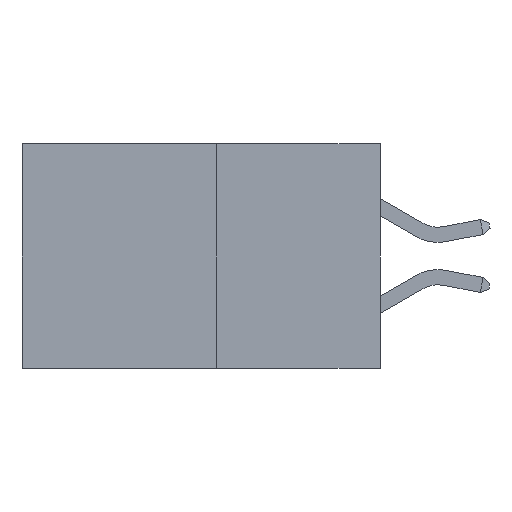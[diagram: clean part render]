
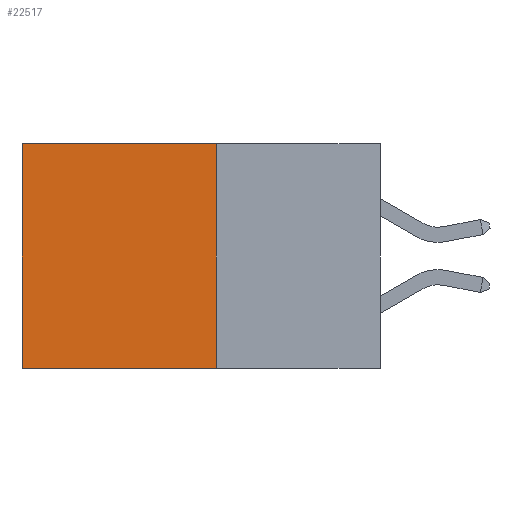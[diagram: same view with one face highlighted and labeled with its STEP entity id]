
A CAD part, left-side view. The second image highlights one B-rep face of the part: STEP entity #22517.
In plain terms, the highlighted planar face has unit normal (-1, 0, 0).
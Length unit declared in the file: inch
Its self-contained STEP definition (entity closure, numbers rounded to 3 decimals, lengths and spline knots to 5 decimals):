
#89 = LINE ( 'NONE', #22665, #4940 ) ;
#749 = EDGE_CURVE ( 'NONE', #18673, #10281, #4809, .T. ) ;
#1871 = ORIENTED_EDGE ( 'NONE', *, *, #24266, .F. ) ;
#1953 = DIRECTION ( 'NONE',  ( 0., 1., 0. ) ) ;
#2488 = CARTESIAN_POINT ( 'NONE',  ( 0.277, 0.27, -0.37 ) ) ;
#2747 = CARTESIAN_POINT ( 'NONE',  ( 0.277, 0.59, -0.37 ) ) ;
#3025 = EDGE_LOOP ( 'NONE', ( #8569, #1871, #23358, #18599 ) ) ;
#4348 = EDGE_CURVE ( 'NONE', #9320, #18673, #89, .T. ) ;
#4773 = VERTEX_POINT ( 'NONE', #17671 ) ;
#4809 = LINE ( 'NONE', #6474, #10126 ) ;
#4938 = DIRECTION ( 'NONE',  ( 0., 0., -1. ) ) ;
#4940 = VECTOR ( 'NONE', #22587, 39.37008 ) ;
#5736 = FACE_OUTER_BOUND ( 'NONE', #3025, .T. ) ;
#5994 = AXIS2_PLACEMENT_3D ( 'NONE', #2488, #16429, #4938 ) ;
#6474 = CARTESIAN_POINT ( 'NONE',  ( 0.277, 0.59, -0.37 ) ) ;
#7237 = DIRECTION ( 'NONE',  ( 0., 0., -1. ) ) ;
#8030 = VECTOR ( 'NONE', #20926, 39.37008 ) ;
#8569 = ORIENTED_EDGE ( 'NONE', *, *, #749, .T. ) ;
#8670 = LINE ( 'NONE', #11082, #8030 ) ;
#9320 = VERTEX_POINT ( 'NONE', #23881 ) ;
#10126 = VECTOR ( 'NONE', #7237, 39.37008 ) ;
#10281 = VERTEX_POINT ( 'NONE', #2747 ) ;
#11082 = CARTESIAN_POINT ( 'NONE',  ( 0.277, 0.27, -0.37 ) ) ;
#13552 = EDGE_CURVE ( 'NONE', #9320, #4773, #8670, .T. ) ;
#16429 = DIRECTION ( 'NONE',  ( 1., 0., 0. ) ) ;
#17671 = CARTESIAN_POINT ( 'NONE',  ( 0.277, 0.27, -0.37 ) ) ;
#18358 = PLANE ( 'NONE',  #5994 ) ;
#18455 = CARTESIAN_POINT ( 'NONE',  ( 0.277, 0.59, 0. ) ) ;
#18599 = ORIENTED_EDGE ( 'NONE', *, *, #4348, .T. ) ;
#18673 = VERTEX_POINT ( 'NONE', #18455 ) ;
#20926 = DIRECTION ( 'NONE',  ( 0., 0., -1. ) ) ;
#22425 = LINE ( 'NONE', #25705, #23466 ) ;
#22517 = ADVANCED_FACE ( 'NONE', ( #5736 ), #18358, .F. ) ;
#22587 = DIRECTION ( 'NONE',  ( 0., 1., 0. ) ) ;
#22665 = CARTESIAN_POINT ( 'NONE',  ( 0.277, 0.27, 0. ) ) ;
#23358 = ORIENTED_EDGE ( 'NONE', *, *, #13552, .F. ) ;
#23466 = VECTOR ( 'NONE', #1953, 39.37008 ) ;
#23881 = CARTESIAN_POINT ( 'NONE',  ( 0.277, 0.27, 0. ) ) ;
#24266 = EDGE_CURVE ( 'NONE', #4773, #10281, #22425, .T. ) ;
#25705 = CARTESIAN_POINT ( 'NONE',  ( 0.277, 0.27, -0.37 ) ) ;
